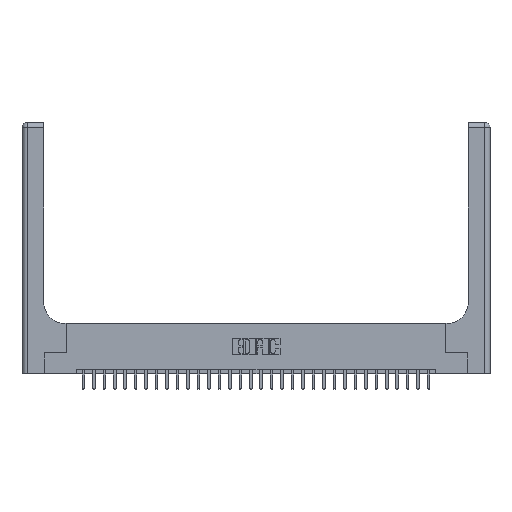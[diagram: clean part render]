
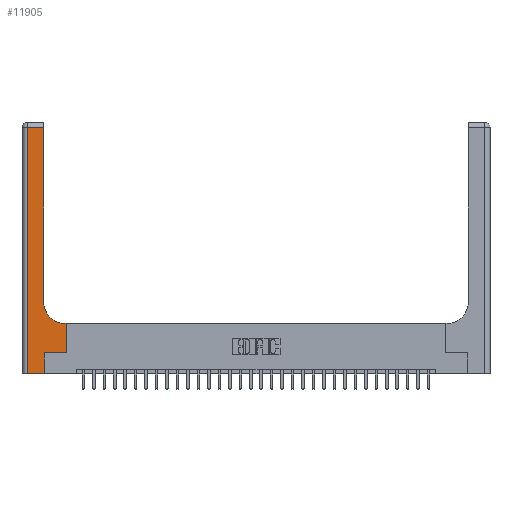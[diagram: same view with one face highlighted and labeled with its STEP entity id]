
A CAD part, top view. The second image highlights one B-rep face of the part: STEP entity #11905.
In plain terms, the highlighted planar face has unit normal (0, 0, 1).
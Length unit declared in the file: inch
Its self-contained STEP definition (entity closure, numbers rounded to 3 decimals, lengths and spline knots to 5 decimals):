
#405 = CARTESIAN_POINT ( 'NONE',  ( 0., 0., 0.37 ) ) ;
#532 = ORIENTED_EDGE ( 'NONE', *, *, #5386, .T. ) ;
#2223 = CARTESIAN_POINT ( 'NONE',  ( 0.26, 0.6, 0.37 ) ) ;
#2743 = ORIENTED_EDGE ( 'NONE', *, *, #16592, .T. ) ;
#3228 = EDGE_CURVE ( 'NONE', #18972, #11384, #11933, .T. ) ;
#3378 = CIRCLE ( 'NONE', #24405, 0.25 ) ;
#3494 = CARTESIAN_POINT ( 'NONE',  ( 0.06, 0., 0.37 ) ) ;
#4313 = VECTOR ( 'NONE', #5222, 39.37008 ) ;
#4511 = EDGE_CURVE ( 'NONE', #28392, #11071, #11397, .T. ) ;
#5222 = DIRECTION ( 'NONE',  ( 0., 1., 0. ) ) ;
#5386 = EDGE_CURVE ( 'NONE', #21755, #21683, #22418, .T. ) ;
#6114 = VECTOR ( 'NONE', #14212, 39.37008 ) ;
#6241 = CARTESIAN_POINT ( 'NONE',  ( 0.265, 0., 0.37 ) ) ;
#6354 = VECTOR ( 'NONE', #17838, 39.37008 ) ;
#6822 = CARTESIAN_POINT ( 'NONE',  ( 0.06, 3., 0.37 ) ) ;
#6919 = VERTEX_POINT ( 'NONE', #11973 ) ;
#7428 = AXIS2_PLACEMENT_3D ( 'NONE', #25793, #14631, #12416 ) ;
#7933 = CARTESIAN_POINT ( 'NONE',  ( 0.265, 0.25, 0.37 ) ) ;
#8012 = ORIENTED_EDGE ( 'NONE', *, *, #16293, .T. ) ;
#8547 = ORIENTED_EDGE ( 'NONE', *, *, #11254, .T. ) ;
#9486 = CARTESIAN_POINT ( 'NONE',  ( 0.265, 0.25, 0.37 ) ) ;
#9501 = ORIENTED_EDGE ( 'NONE', *, *, #3228, .T. ) ;
#9986 = LINE ( 'NONE', #7933, #6114 ) ;
#10716 = LINE ( 'NONE', #15092, #26254 ) ;
#10899 = DIRECTION ( 'NONE',  ( 0., 1., 0. ) ) ;
#11071 = VERTEX_POINT ( 'NONE', #15282 ) ;
#11135 = ORIENTED_EDGE ( 'NONE', *, *, #4511, .T. ) ;
#11158 = DIRECTION ( 'NONE',  ( -1., 0., 0. ) ) ;
#11254 = EDGE_CURVE ( 'NONE', #6919, #28392, #26887, .T. ) ;
#11384 = VERTEX_POINT ( 'NONE', #20699 ) ;
#11397 = LINE ( 'NONE', #405, #6354 ) ;
#11905 = ADVANCED_FACE ( 'NONE', ( #17134 ), #26239, .F. ) ;
#11933 = LINE ( 'NONE', #22486, #4313 ) ;
#11973 = CARTESIAN_POINT ( 'NONE',  ( 0.06, 2.94, 0.37 ) ) ;
#12392 = EDGE_CURVE ( 'NONE', #11071, #27422, #23792, .T. ) ;
#12416 = DIRECTION ( 'NONE',  ( -1., 0., 0. ) ) ;
#12988 = EDGE_CURVE ( 'NONE', #11384, #20423, #20068, .T. ) ;
#13377 = VECTOR ( 'NONE', #25067, 39.37008 ) ;
#14139 = CARTESIAN_POINT ( 'NONE',  ( 0.51, 0.6, 0.37 ) ) ;
#14212 = DIRECTION ( 'NONE',  ( 1., 0., 0. ) ) ;
#14631 = DIRECTION ( 'NONE',  ( 0., 0., -1. ) ) ;
#15092 = CARTESIAN_POINT ( 'NONE',  ( 0., 2.94, 0.37 ) ) ;
#15282 = CARTESIAN_POINT ( 'NONE',  ( 0.265, 0., 0.37 ) ) ;
#16029 = DIRECTION ( 'NONE',  ( 0., 0., -1. ) ) ;
#16217 = ORIENTED_EDGE ( 'NONE', *, *, #12988, .T. ) ;
#16293 = EDGE_CURVE ( 'NONE', #27422, #18972, #9986, .T. ) ;
#16495 = CARTESIAN_POINT ( 'NONE',  ( 0.26, 0.85, 0.37 ) ) ;
#16592 = EDGE_CURVE ( 'NONE', #21683, #6919, #10716, .T. ) ;
#16813 = VECTOR ( 'NONE', #11158, 39.37008 ) ;
#17134 = FACE_OUTER_BOUND ( 'NONE', #19300, .T. ) ;
#17630 = DIRECTION ( 'NONE',  ( 0., -1., 0. ) ) ;
#17838 = DIRECTION ( 'NONE',  ( 1., 0., 0. ) ) ;
#18972 = VERTEX_POINT ( 'NONE', #22600 ) ;
#19300 = EDGE_LOOP ( 'NONE', ( #532, #2743, #8547, #11135, #26862, #8012, #9501, #16217, #28219 ) ) ;
#20068 = LINE ( 'NONE', #2223, #16813 ) ;
#20423 = VERTEX_POINT ( 'NONE', #14139 ) ;
#20662 = CARTESIAN_POINT ( 'NONE',  ( 0.26, 3., 0.37 ) ) ;
#20699 = CARTESIAN_POINT ( 'NONE',  ( 0.528, 0.6, 0.37 ) ) ;
#21683 = VERTEX_POINT ( 'NONE', #25014 ) ;
#21755 = VERTEX_POINT ( 'NONE', #16495 ) ;
#21841 = VECTOR ( 'NONE', #17630, 39.37008 ) ;
#22418 = LINE ( 'NONE', #20662, #13377 ) ;
#22486 = CARTESIAN_POINT ( 'NONE',  ( 0.528, 0.25, 0.37 ) ) ;
#22600 = CARTESIAN_POINT ( 'NONE',  ( 0.528, 0.25, 0.37 ) ) ;
#22747 = DIRECTION ( 'NONE',  ( 1., 0., 0. ) ) ;
#23792 = LINE ( 'NONE', #6241, #26050 ) ;
#24405 = AXIS2_PLACEMENT_3D ( 'NONE', #25122, #16029, #22747 ) ;
#25014 = CARTESIAN_POINT ( 'NONE',  ( 0.26, 2.94, 0.37 ) ) ;
#25067 = DIRECTION ( 'NONE',  ( 0., 1., 0. ) ) ;
#25122 = CARTESIAN_POINT ( 'NONE',  ( 0.51, 0.85, 0.37 ) ) ;
#25793 = CARTESIAN_POINT ( 'NONE',  ( 0., 3., 0.37 ) ) ;
#26050 = VECTOR ( 'NONE', #10899, 39.37008 ) ;
#26239 = PLANE ( 'NONE',  #7428 ) ;
#26254 = VECTOR ( 'NONE', #28327, 39.37008 ) ;
#26862 = ORIENTED_EDGE ( 'NONE', *, *, #12392, .T. ) ;
#26887 = LINE ( 'NONE', #6822, #21841 ) ;
#27422 = VERTEX_POINT ( 'NONE', #9486 ) ;
#27904 = EDGE_CURVE ( 'NONE', #20423, #21755, #3378, .T. ) ;
#28219 = ORIENTED_EDGE ( 'NONE', *, *, #27904, .T. ) ;
#28327 = DIRECTION ( 'NONE',  ( -1., 0., 0. ) ) ;
#28392 = VERTEX_POINT ( 'NONE', #3494 ) ;
